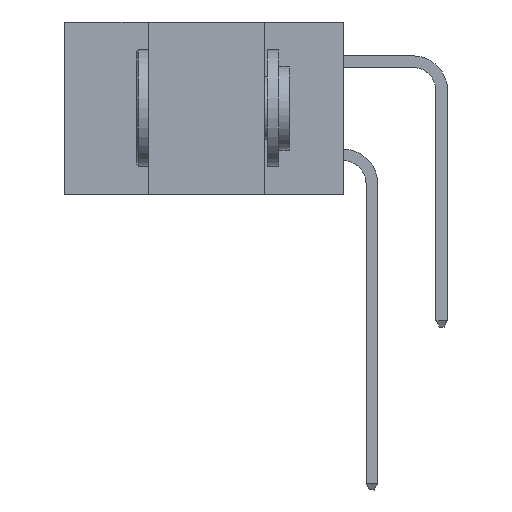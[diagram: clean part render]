
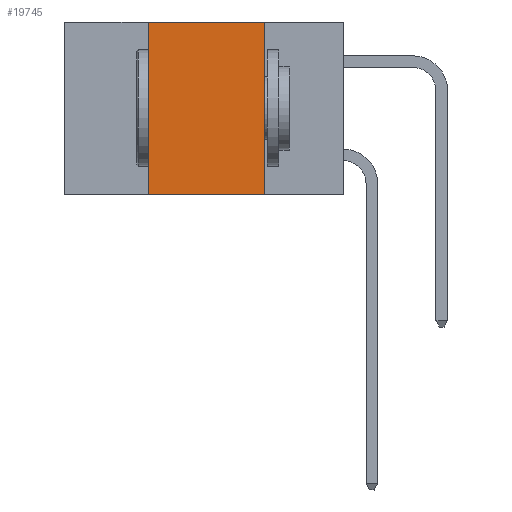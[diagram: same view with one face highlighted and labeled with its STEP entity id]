
A CAD part, left-side view. The second image highlights one B-rep face of the part: STEP entity #19745.
In plain terms, the highlighted planar face has unit normal (-1, 0, 0).
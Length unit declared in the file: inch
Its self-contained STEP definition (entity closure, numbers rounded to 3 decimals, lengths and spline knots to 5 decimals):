
#1007 = DIRECTION ( 'NONE',  ( 0., -1., 0. ) ) ;
#1170 = LINE ( 'NONE', #15139, #4886 ) ;
#2371 = CARTESIAN_POINT ( 'NONE',  ( 0., 0.17, -0.37 ) ) ;
#2503 = DIRECTION ( 'NONE',  ( 0., 0., 1. ) ) ;
#2552 = VERTEX_POINT ( 'NONE', #6685 ) ;
#3264 = EDGE_CURVE ( 'NONE', #7558, #20161, #14271, .T. ) ;
#3409 = VECTOR ( 'NONE', #2503, 39.37008 ) ;
#4083 = CARTESIAN_POINT ( 'NONE',  ( 0., 0.42, 0. ) ) ;
#4886 = VECTOR ( 'NONE', #11953, 39.37008 ) ;
#5331 = VECTOR ( 'NONE', #1007, 39.37008 ) ;
#6515 = EDGE_CURVE ( 'NONE', #7558, #2552, #8177, .T. ) ;
#6553 = AXIS2_PLACEMENT_3D ( 'NONE', #17174, #18636, #9272 ) ;
#6685 = CARTESIAN_POINT ( 'NONE',  ( 0., 0.42, 0. ) ) ;
#7558 = VERTEX_POINT ( 'NONE', #18105 ) ;
#7593 = EDGE_CURVE ( 'NONE', #18966, #20161, #1170, .T. ) ;
#8177 = LINE ( 'NONE', #4083, #3409 ) ;
#8646 = EDGE_LOOP ( 'NONE', ( #19683, #10592, #13791, #12422 ) ) ;
#9272 = DIRECTION ( 'NONE',  ( 0., 0., -1. ) ) ;
#10592 = ORIENTED_EDGE ( 'NONE', *, *, #14993, .F. ) ;
#11953 = DIRECTION ( 'NONE',  ( 0., 0., -1. ) ) ;
#12422 = ORIENTED_EDGE ( 'NONE', *, *, #3264, .T. ) ;
#13074 = CARTESIAN_POINT ( 'NONE',  ( 0., 0.17, 0. ) ) ;
#13791 = ORIENTED_EDGE ( 'NONE', *, *, #6515, .F. ) ;
#14271 = LINE ( 'NONE', #15026, #5331 ) ;
#14496 = CARTESIAN_POINT ( 'NONE',  ( 0., 0.6, 0. ) ) ;
#14993 = EDGE_CURVE ( 'NONE', #2552, #18966, #19640, .T. ) ;
#15026 = CARTESIAN_POINT ( 'NONE',  ( 0., 0.6, -0.37 ) ) ;
#15139 = CARTESIAN_POINT ( 'NONE',  ( 0., 0.17, 0. ) ) ;
#15559 = PLANE ( 'NONE',  #6553 ) ;
#15617 = VECTOR ( 'NONE', #16085, 39.37008 ) ;
#16085 = DIRECTION ( 'NONE',  ( 0., -1., 0. ) ) ;
#16733 = FACE_OUTER_BOUND ( 'NONE', #8646, .T. ) ;
#17174 = CARTESIAN_POINT ( 'NONE',  ( 0., 0.6, 0. ) ) ;
#18105 = CARTESIAN_POINT ( 'NONE',  ( 0., 0.42, -0.37 ) ) ;
#18636 = DIRECTION ( 'NONE',  ( 1., 0., 0. ) ) ;
#18966 = VERTEX_POINT ( 'NONE', #13074 ) ;
#19640 = LINE ( 'NONE', #14496, #15617 ) ;
#19683 = ORIENTED_EDGE ( 'NONE', *, *, #7593, .F. ) ;
#19745 = ADVANCED_FACE ( 'NONE', ( #16733 ), #15559, .F. ) ;
#20161 = VERTEX_POINT ( 'NONE', #2371 ) ;
